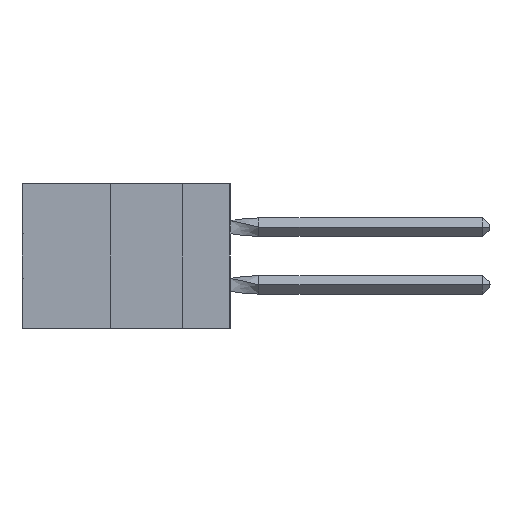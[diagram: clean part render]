
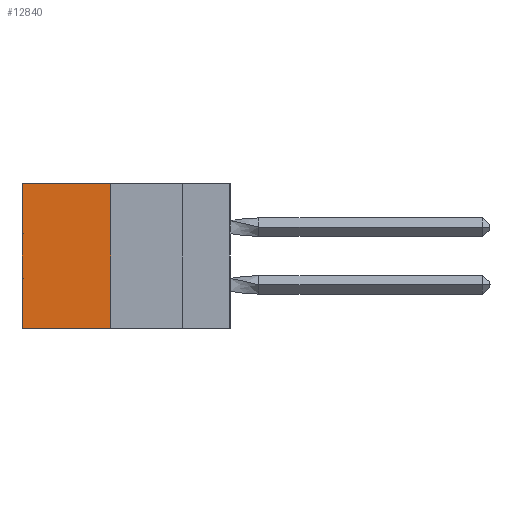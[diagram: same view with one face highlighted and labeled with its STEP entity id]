
A CAD part, left-side view. The second image highlights one B-rep face of the part: STEP entity #12840.
In plain terms, the highlighted planar face has unit normal (-1, 0, 0).
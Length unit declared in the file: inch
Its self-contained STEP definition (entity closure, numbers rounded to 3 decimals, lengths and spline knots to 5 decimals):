
#1725 = VECTOR ( 'NONE', #35073, 39.37008 ) ;
#2116 = EDGE_LOOP ( 'NONE', ( #44064, #46269, #12298, #29139 ) ) ;
#2946 = EDGE_CURVE ( 'NONE', #33276, #42415, #27513, .T. ) ;
#4645 = EDGE_CURVE ( 'NONE', #42415, #15337, #22934, .T. ) ;
#7842 = CARTESIAN_POINT ( 'NONE',  ( 0.305, 0.72, 0. ) ) ;
#8010 = CARTESIAN_POINT ( 'NONE',  ( 0.305, 0.413, -0.5 ) ) ;
#8781 = LINE ( 'NONE', #10559, #34620 ) ;
#10027 = FACE_OUTER_BOUND ( 'NONE', #2116, .T. ) ;
#10559 = CARTESIAN_POINT ( 'NONE',  ( 0.305, 0.72, -0.5 ) ) ;
#12298 = ORIENTED_EDGE ( 'NONE', *, *, #2946, .F. ) ;
#12840 = ADVANCED_FACE ( 'NONE', ( #10027 ), #41277, .F. ) ;
#15196 = CARTESIAN_POINT ( 'NONE',  ( 0.305, 0.413, -0.5 ) ) ;
#15337 = VERTEX_POINT ( 'NONE', #22502 ) ;
#19661 = DIRECTION ( 'NONE',  ( 0., 1., 0. ) ) ;
#20962 = CARTESIAN_POINT ( 'NONE',  ( 0.305, 0.413, -0.5 ) ) ;
#22462 = DIRECTION ( 'NONE',  ( 0., 0., -1. ) ) ;
#22502 = CARTESIAN_POINT ( 'NONE',  ( 0.305, 0.72, -0.5 ) ) ;
#22934 = LINE ( 'NONE', #20962, #40856 ) ;
#22989 = EDGE_CURVE ( 'NONE', #33276, #29701, #33021, .T. ) ;
#25452 = DIRECTION ( 'NONE',  ( 0., 0., -1. ) ) ;
#27513 = LINE ( 'NONE', #38477, #1725 ) ;
#29139 = ORIENTED_EDGE ( 'NONE', *, *, #22989, .T. ) ;
#29690 = CARTESIAN_POINT ( 'NONE',  ( 0.305, 0.413, 0. ) ) ;
#29701 = VERTEX_POINT ( 'NONE', #7842 ) ;
#30753 = VECTOR ( 'NONE', #19661, 39.37008 ) ;
#31938 = AXIS2_PLACEMENT_3D ( 'NONE', #15196, #40278, #22462 ) ;
#33021 = LINE ( 'NONE', #43872, #30753 ) ;
#33276 = VERTEX_POINT ( 'NONE', #29690 ) ;
#34620 = VECTOR ( 'NONE', #25452, 39.37008 ) ;
#35073 = DIRECTION ( 'NONE',  ( 0., 0., -1. ) ) ;
#38477 = CARTESIAN_POINT ( 'NONE',  ( 0.305, 0.413, -0.5 ) ) ;
#40278 = DIRECTION ( 'NONE',  ( 1., 0., 0. ) ) ;
#40856 = VECTOR ( 'NONE', #45952, 39.37008 ) ;
#41277 = PLANE ( 'NONE',  #31938 ) ;
#42348 = EDGE_CURVE ( 'NONE', #29701, #15337, #8781, .T. ) ;
#42415 = VERTEX_POINT ( 'NONE', #8010 ) ;
#43872 = CARTESIAN_POINT ( 'NONE',  ( 0.305, 0.413, 0. ) ) ;
#44064 = ORIENTED_EDGE ( 'NONE', *, *, #42348, .T. ) ;
#45952 = DIRECTION ( 'NONE',  ( 0., 1., 0. ) ) ;
#46269 = ORIENTED_EDGE ( 'NONE', *, *, #4645, .F. ) ;
